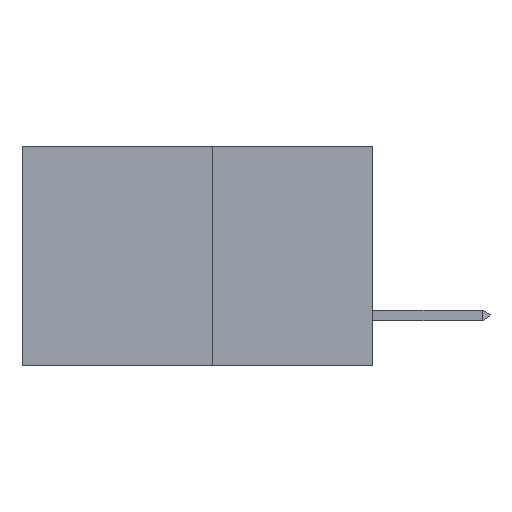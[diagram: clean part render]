
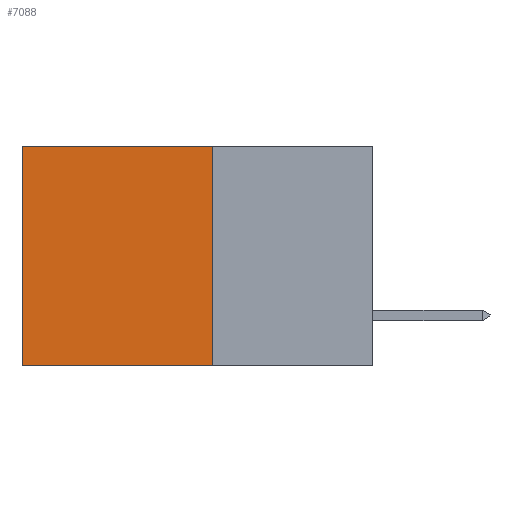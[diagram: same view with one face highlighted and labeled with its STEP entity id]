
A CAD part, left-side view. The second image highlights one B-rep face of the part: STEP entity #7088.
In plain terms, the highlighted planar face has unit normal (-1, 0, 0).
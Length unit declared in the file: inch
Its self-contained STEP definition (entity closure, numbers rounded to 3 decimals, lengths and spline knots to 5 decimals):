
#1165 = CARTESIAN_POINT ( 'NONE',  ( 0.277, 0.27, -0.37 ) ) ;
#2357 = VERTEX_POINT ( 'NONE', #2938 ) ;
#2938 = CARTESIAN_POINT ( 'NONE',  ( 0.277, 0.27, 0. ) ) ;
#3634 = DIRECTION ( 'NONE',  ( 0., 0., -1. ) ) ;
#4242 = CARTESIAN_POINT ( 'NONE',  ( 0.277, 0.59, 0. ) ) ;
#5573 = VECTOR ( 'NONE', #9845, 39.37008 ) ;
#7013 = CARTESIAN_POINT ( 'NONE',  ( 0.277, 0.27, -0.37 ) ) ;
#7088 = ADVANCED_FACE ( 'NONE', ( #26769 ), #24921, .F. ) ;
#7749 = ORIENTED_EDGE ( 'NONE', *, *, #27290, .T. ) ;
#8647 = VERTEX_POINT ( 'NONE', #9314 ) ;
#8660 = CARTESIAN_POINT ( 'NONE',  ( 0.277, 0.27, 0. ) ) ;
#9314 = CARTESIAN_POINT ( 'NONE',  ( 0.277, 0.59, -0.37 ) ) ;
#9383 = DIRECTION ( 'NONE',  ( 0., 0., -1. ) ) ;
#9802 = VECTOR ( 'NONE', #27552, 39.37008 ) ;
#9845 = DIRECTION ( 'NONE',  ( 0., 1., 0. ) ) ;
#10820 = LINE ( 'NONE', #7013, #22685 ) ;
#11273 = ORIENTED_EDGE ( 'NONE', *, *, #22719, .F. ) ;
#11633 = CARTESIAN_POINT ( 'NONE',  ( 0.277, 0.27, -0.37 ) ) ;
#13818 = EDGE_LOOP ( 'NONE', ( #7749, #11273, #18448, #22327 ) ) ;
#15370 = DIRECTION ( 'NONE',  ( 0., 0., -1. ) ) ;
#16083 = LINE ( 'NONE', #8660, #9802 ) ;
#17882 = DIRECTION ( 'NONE',  ( 1., 0., 0. ) ) ;
#18448 = ORIENTED_EDGE ( 'NONE', *, *, #29916, .F. ) ;
#19241 = CARTESIAN_POINT ( 'NONE',  ( 0.277, 0.27, -0.37 ) ) ;
#21310 = LINE ( 'NONE', #22454, #26845 ) ;
#22327 = ORIENTED_EDGE ( 'NONE', *, *, #27894, .T. ) ;
#22454 = CARTESIAN_POINT ( 'NONE',  ( 0.277, 0.59, -0.37 ) ) ;
#22685 = VECTOR ( 'NONE', #9383, 39.37008 ) ;
#22719 = EDGE_CURVE ( 'NONE', #25697, #8647, #30650, .T. ) ;
#23870 = AXIS2_PLACEMENT_3D ( 'NONE', #1165, #17882, #3634 ) ;
#24921 = PLANE ( 'NONE',  #23870 ) ;
#25697 = VERTEX_POINT ( 'NONE', #11633 ) ;
#26769 = FACE_OUTER_BOUND ( 'NONE', #13818, .T. ) ;
#26845 = VECTOR ( 'NONE', #15370, 39.37008 ) ;
#27290 = EDGE_CURVE ( 'NONE', #27980, #8647, #21310, .T. ) ;
#27552 = DIRECTION ( 'NONE',  ( 0., 1., 0. ) ) ;
#27894 = EDGE_CURVE ( 'NONE', #2357, #27980, #16083, .T. ) ;
#27980 = VERTEX_POINT ( 'NONE', #4242 ) ;
#29916 = EDGE_CURVE ( 'NONE', #2357, #25697, #10820, .T. ) ;
#30650 = LINE ( 'NONE', #19241, #5573 ) ;
